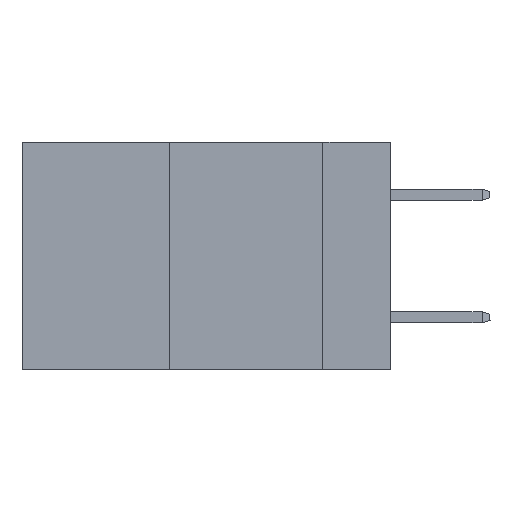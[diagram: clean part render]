
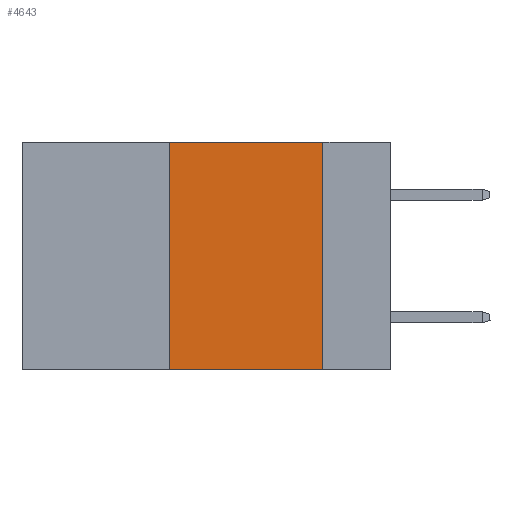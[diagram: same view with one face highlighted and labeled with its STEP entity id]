
A CAD part, left-side view. The second image highlights one B-rep face of the part: STEP entity #4643.
In plain terms, the highlighted planar face has unit normal (-1, 0, 0).
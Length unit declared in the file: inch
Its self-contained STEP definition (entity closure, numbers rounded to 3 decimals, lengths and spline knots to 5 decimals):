
#992 = VECTOR ( 'NONE', #4291, 39.37008 ) ;
#995 = EDGE_CURVE ( 'NONE', #2759, #15661, #3111, .T. ) ;
#1011 = VECTOR ( 'NONE', #14678, 39.37008 ) ;
#1449 = VERTEX_POINT ( 'NONE', #10152 ) ;
#1590 = LINE ( 'NONE', #3001, #5537 ) ;
#2715 = CARTESIAN_POINT ( 'NONE',  ( 0., 0.36, -0.37 ) ) ;
#2759 = VERTEX_POINT ( 'NONE', #2715 ) ;
#2897 = CARTESIAN_POINT ( 'NONE',  ( 0., 0.11, 0. ) ) ;
#3001 = CARTESIAN_POINT ( 'NONE',  ( 0., 0.36, 0. ) ) ;
#3111 = LINE ( 'NONE', #20725, #992 ) ;
#3808 = ORIENTED_EDGE ( 'NONE', *, *, #995, .T. ) ;
#4108 = ORIENTED_EDGE ( 'NONE', *, *, #7522, .F. ) ;
#4291 = DIRECTION ( 'NONE',  ( 0., -1., 0. ) ) ;
#4593 = DIRECTION ( 'NONE',  ( 0., -1., 0. ) ) ;
#4630 = DIRECTION ( 'NONE',  ( 0., 0., -1. ) ) ;
#4643 = ADVANCED_FACE ( 'NONE', ( #10416 ), #7988, .F. ) ;
#4695 = DIRECTION ( 'NONE',  ( 0., 0., 1. ) ) ;
#5449 = EDGE_CURVE ( 'NONE', #2759, #1449, #1590, .T. ) ;
#5537 = VECTOR ( 'NONE', #4695, 39.37008 ) ;
#6573 = LINE ( 'NONE', #19903, #1011 ) ;
#7522 = EDGE_CURVE ( 'NONE', #1449, #15452, #8121, .T. ) ;
#7940 = CARTESIAN_POINT ( 'NONE',  ( 0., 0.6, 0. ) ) ;
#7988 = PLANE ( 'NONE',  #8892 ) ;
#8121 = LINE ( 'NONE', #7940, #9980 ) ;
#8892 = AXIS2_PLACEMENT_3D ( 'NONE', #9464, #21632, #4630 ) ;
#9464 = CARTESIAN_POINT ( 'NONE',  ( 0., 0.6, 0. ) ) ;
#9980 = VECTOR ( 'NONE', #4593, 39.37008 ) ;
#10135 = ORIENTED_EDGE ( 'NONE', *, *, #5449, .F. ) ;
#10152 = CARTESIAN_POINT ( 'NONE',  ( 0., 0.36, 0. ) ) ;
#10416 = FACE_OUTER_BOUND ( 'NONE', #18337, .T. ) ;
#14678 = DIRECTION ( 'NONE',  ( 0., 0., -1. ) ) ;
#15452 = VERTEX_POINT ( 'NONE', #2897 ) ;
#15661 = VERTEX_POINT ( 'NONE', #21716 ) ;
#15792 = EDGE_CURVE ( 'NONE', #15452, #15661, #6573, .T. ) ;
#18337 = EDGE_LOOP ( 'NONE', ( #21801, #4108, #10135, #3808 ) ) ;
#19903 = CARTESIAN_POINT ( 'NONE',  ( 0., 0.11, 0. ) ) ;
#20725 = CARTESIAN_POINT ( 'NONE',  ( 0., 0.6, -0.37 ) ) ;
#21632 = DIRECTION ( 'NONE',  ( 1., 0., 0. ) ) ;
#21716 = CARTESIAN_POINT ( 'NONE',  ( 0., 0.11, -0.37 ) ) ;
#21801 = ORIENTED_EDGE ( 'NONE', *, *, #15792, .F. ) ;
